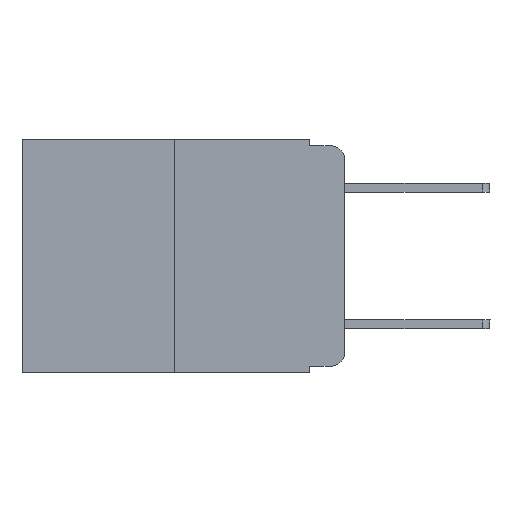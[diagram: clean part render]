
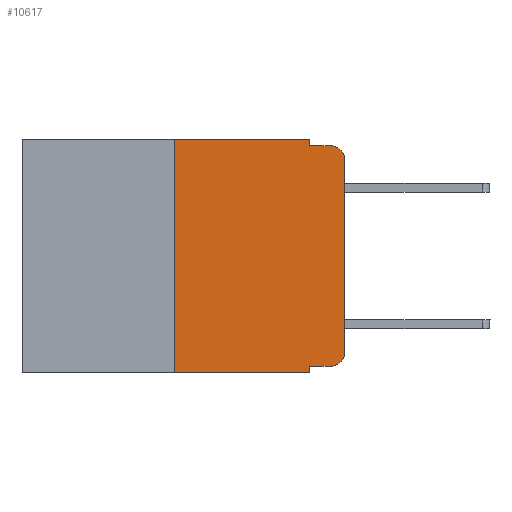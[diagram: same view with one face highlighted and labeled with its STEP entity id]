
A CAD part, left-side view. The second image highlights one B-rep face of the part: STEP entity #10617.
In plain terms, the highlighted planar face has unit normal (-1, 0, 0).
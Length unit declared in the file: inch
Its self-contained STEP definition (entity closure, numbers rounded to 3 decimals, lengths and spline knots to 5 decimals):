
#640 = CARTESIAN_POINT ( 'NONE',  ( 0., 0.051, -0.333 ) ) ;
#782 = CARTESIAN_POINT ( 'NONE',  ( 0., 0.473, 0. ) ) ;
#862 = DIRECTION ( 'NONE',  ( 1., 0., 0. ) ) ;
#1216 = VECTOR ( 'NONE', #8825, 39.37008 ) ;
#1659 = DIRECTION ( 'NONE',  ( -1., 0., 0. ) ) ;
#1700 = EDGE_CURVE ( 'NONE', #10930, #5578, #6975, .T. ) ;
#1787 = PLANE ( 'NONE',  #4780 ) ;
#1911 = CARTESIAN_POINT ( 'NONE',  ( 0., 0.473, -0.343 ) ) ;
#2079 = CARTESIAN_POINT ( 'NONE',  ( 0., 0.051, 0. ) ) ;
#2331 = ORIENTED_EDGE ( 'NONE', *, *, #6024, .F. ) ;
#2347 = VERTEX_POINT ( 'NONE', #11823 ) ;
#2612 = LINE ( 'NONE', #3693, #9150 ) ;
#2637 = DIRECTION ( 'NONE',  ( 0., 0., -1. ) ) ;
#2651 = AXIS2_PLACEMENT_3D ( 'NONE', #7542, #1659, #2637 ) ;
#3094 = VECTOR ( 'NONE', #8557, 39.37008 ) ;
#3123 = DIRECTION ( 'NONE',  ( 0., -1., 0. ) ) ;
#3207 = VERTEX_POINT ( 'NONE', #9031 ) ;
#3693 = CARTESIAN_POINT ( 'NONE',  ( 0., 0.051, 0. ) ) ;
#3831 = LINE ( 'NONE', #640, #11229 ) ;
#3858 = VECTOR ( 'NONE', #6881, 39.37008 ) ;
#4159 = EDGE_CURVE ( 'NONE', #6983, #5557, #12609, .T. ) ;
#4238 = CARTESIAN_POINT ( 'NONE',  ( 0., 0.02, -0.313 ) ) ;
#4447 = EDGE_CURVE ( 'NONE', #3207, #9630, #5911, .T. ) ;
#4575 = EDGE_CURVE ( 'NONE', #5578, #9090, #11393, .T. ) ;
#4739 = AXIS2_PLACEMENT_3D ( 'NONE', #4238, #5328, #11241 ) ;
#4780 = AXIS2_PLACEMENT_3D ( 'NONE', #11822, #862, #4800 ) ;
#4800 = DIRECTION ( 'NONE',  ( 0., 0., -1. ) ) ;
#5100 = LINE ( 'NONE', #12154, #5390 ) ;
#5136 = EDGE_CURVE ( 'NONE', #2347, #9090, #12561, .T. ) ;
#5328 = DIRECTION ( 'NONE',  ( -1., 0., 0. ) ) ;
#5390 = VECTOR ( 'NONE', #10055, 39.37008 ) ;
#5436 = CARTESIAN_POINT ( 'NONE',  ( 0., 0.02, -0.333 ) ) ;
#5557 = VERTEX_POINT ( 'NONE', #12448 ) ;
#5578 = VERTEX_POINT ( 'NONE', #11493 ) ;
#5911 = LINE ( 'NONE', #1911, #3858 ) ;
#6024 = EDGE_CURVE ( 'NONE', #11252, #9630, #2612, .T. ) ;
#6102 = ORIENTED_EDGE ( 'NONE', *, *, #7882, .T. ) ;
#6160 = CARTESIAN_POINT ( 'NONE',  ( 0., 0.051, -0.333 ) ) ;
#6517 = ORIENTED_EDGE ( 'NONE', *, *, #4447, .T. ) ;
#6538 = LINE ( 'NONE', #782, #12445 ) ;
#6770 = ORIENTED_EDGE ( 'NONE', *, *, #4159, .T. ) ;
#6881 = DIRECTION ( 'NONE',  ( 0., -1., 0. ) ) ;
#6975 = LINE ( 'NONE', #2079, #1216 ) ;
#6983 = VERTEX_POINT ( 'NONE', #5436 ) ;
#7085 = CARTESIAN_POINT ( 'NONE',  ( 0., 0.02, -0.01 ) ) ;
#7542 = CARTESIAN_POINT ( 'NONE',  ( 0., 0.02, -0.03 ) ) ;
#7575 = DIRECTION ( 'NONE',  ( 0., 0., -1. ) ) ;
#7772 = DIRECTION ( 'NONE',  ( 0., -1., 0. ) ) ;
#7882 = EDGE_CURVE ( 'NONE', #5557, #2347, #12550, .T. ) ;
#8384 = ORIENTED_EDGE ( 'NONE', *, *, #4575, .F. ) ;
#8557 = DIRECTION ( 'NONE',  ( 0., 0., 1. ) ) ;
#8616 = ORIENTED_EDGE ( 'NONE', *, *, #9920, .F. ) ;
#8734 = ORIENTED_EDGE ( 'NONE', *, *, #11115, .T. ) ;
#8825 = DIRECTION ( 'NONE',  ( 0., 0., -1. ) ) ;
#9031 = CARTESIAN_POINT ( 'NONE',  ( 0., 0.25, -0.343 ) ) ;
#9090 = VERTEX_POINT ( 'NONE', #7085 ) ;
#9150 = VECTOR ( 'NONE', #7575, 39.37008 ) ;
#9270 = VECTOR ( 'NONE', #3123, 39.37008 ) ;
#9395 = CARTESIAN_POINT ( 'NONE',  ( 0., 0.25, 0. ) ) ;
#9626 = DIRECTION ( 'NONE',  ( 0., -1., 0. ) ) ;
#9630 = VERTEX_POINT ( 'NONE', #12366 ) ;
#9722 = ORIENTED_EDGE ( 'NONE', *, *, #1700, .F. ) ;
#9733 = EDGE_LOOP ( 'NONE', ( #6102, #11638, #8384, #9722, #12474, #8616, #6517, #2331, #8734, #6770 ) ) ;
#9761 = FACE_OUTER_BOUND ( 'NONE', #9733, .T. ) ;
#9920 = EDGE_CURVE ( 'NONE', #3207, #11577, #5100, .T. ) ;
#10055 = DIRECTION ( 'NONE',  ( 0., 0., 1. ) ) ;
#10368 = CARTESIAN_POINT ( 'NONE',  ( 0., 0., 0. ) ) ;
#10617 = ADVANCED_FACE ( 'NONE', ( #9761 ), #1787, .F. ) ;
#10671 = EDGE_CURVE ( 'NONE', #11577, #10930, #6538, .T. ) ;
#10930 = VERTEX_POINT ( 'NONE', #12251 ) ;
#11115 = EDGE_CURVE ( 'NONE', #11252, #6983, #3831, .T. ) ;
#11229 = VECTOR ( 'NONE', #7772, 39.37008 ) ;
#11241 = DIRECTION ( 'NONE',  ( 0., 0., -1. ) ) ;
#11252 = VERTEX_POINT ( 'NONE', #6160 ) ;
#11393 = LINE ( 'NONE', #12006, #9270 ) ;
#11493 = CARTESIAN_POINT ( 'NONE',  ( 0., 0.051, -0.01 ) ) ;
#11577 = VERTEX_POINT ( 'NONE', #9395 ) ;
#11638 = ORIENTED_EDGE ( 'NONE', *, *, #5136, .T. ) ;
#11822 = CARTESIAN_POINT ( 'NONE',  ( 0., 0.473, 0. ) ) ;
#11823 = CARTESIAN_POINT ( 'NONE',  ( 0., 0., -0.03 ) ) ;
#12006 = CARTESIAN_POINT ( 'NONE',  ( 0., 0.051, -0.01 ) ) ;
#12154 = CARTESIAN_POINT ( 'NONE',  ( 0., 0.25, 0. ) ) ;
#12251 = CARTESIAN_POINT ( 'NONE',  ( 0., 0.051, 0. ) ) ;
#12366 = CARTESIAN_POINT ( 'NONE',  ( 0., 0.051, -0.343 ) ) ;
#12445 = VECTOR ( 'NONE', #9626, 39.37008 ) ;
#12448 = CARTESIAN_POINT ( 'NONE',  ( 0., 0., -0.313 ) ) ;
#12474 = ORIENTED_EDGE ( 'NONE', *, *, #10671, .F. ) ;
#12550 = LINE ( 'NONE', #10368, #3094 ) ;
#12561 = CIRCLE ( 'NONE', #2651, 0.02 ) ;
#12609 = CIRCLE ( 'NONE', #4739, 0.02 ) ;
